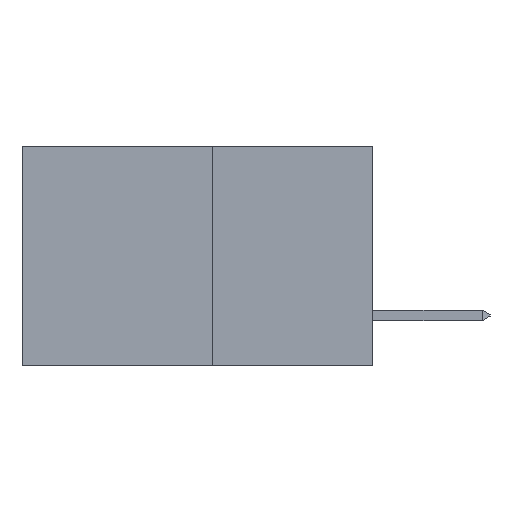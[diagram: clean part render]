
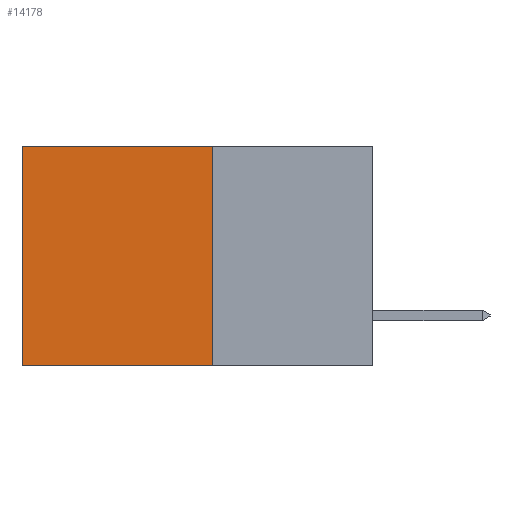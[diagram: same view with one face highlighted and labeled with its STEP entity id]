
A CAD part, left-side view. The second image highlights one B-rep face of the part: STEP entity #14178.
In plain terms, the highlighted planar face has unit normal (-1, 0, 0).
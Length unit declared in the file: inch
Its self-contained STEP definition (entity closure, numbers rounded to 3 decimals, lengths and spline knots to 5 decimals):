
#647 = CARTESIAN_POINT ( 'NONE',  ( 0.277, 0.27, -0.37 ) ) ;
#1127 = DIRECTION ( 'NONE',  ( 0., 0., -1. ) ) ;
#1196 = CARTESIAN_POINT ( 'NONE',  ( 0.277, 0.59, -0.37 ) ) ;
#1388 = VERTEX_POINT ( 'NONE', #10298 ) ;
#2041 = CARTESIAN_POINT ( 'NONE',  ( 0.277, 0.59, -0.37 ) ) ;
#2064 = EDGE_LOOP ( 'NONE', ( #6941, #7075, #2774, #9379 ) ) ;
#2774 = ORIENTED_EDGE ( 'NONE', *, *, #3381, .F. ) ;
#3226 = VERTEX_POINT ( 'NONE', #1196 ) ;
#3381 = EDGE_CURVE ( 'NONE', #1388, #15335, #8486, .T. ) ;
#3581 = DIRECTION ( 'NONE',  ( 0., 0., -1. ) ) ;
#3690 = DIRECTION ( 'NONE',  ( 0., 1., 0. ) ) ;
#3739 = DIRECTION ( 'NONE',  ( 0., 0., -1. ) ) ;
#3917 = VECTOR ( 'NONE', #13736, 39.37008 ) ;
#5325 = LINE ( 'NONE', #15149, #3917 ) ;
#5995 = VECTOR ( 'NONE', #3690, 39.37008 ) ;
#6291 = VERTEX_POINT ( 'NONE', #17651 ) ;
#6637 = EDGE_CURVE ( 'NONE', #6291, #3226, #11202, .T. ) ;
#6914 = LINE ( 'NONE', #14098, #5995 ) ;
#6941 = ORIENTED_EDGE ( 'NONE', *, *, #6637, .T. ) ;
#7075 = ORIENTED_EDGE ( 'NONE', *, *, #7158, .F. ) ;
#7158 = EDGE_CURVE ( 'NONE', #15335, #3226, #5325, .T. ) ;
#7895 = CARTESIAN_POINT ( 'NONE',  ( 0.277, 0.27, -0.37 ) ) ;
#8162 = AXIS2_PLACEMENT_3D ( 'NONE', #647, #12715, #3739 ) ;
#8486 = LINE ( 'NONE', #18847, #11987 ) ;
#9379 = ORIENTED_EDGE ( 'NONE', *, *, #12828, .T. ) ;
#10298 = CARTESIAN_POINT ( 'NONE',  ( 0.277, 0.27, 0. ) ) ;
#10733 = VECTOR ( 'NONE', #3581, 39.37008 ) ;
#11202 = LINE ( 'NONE', #2041, #10733 ) ;
#11987 = VECTOR ( 'NONE', #1127, 39.37008 ) ;
#12715 = DIRECTION ( 'NONE',  ( 1., 0., 0. ) ) ;
#12828 = EDGE_CURVE ( 'NONE', #1388, #6291, #6914, .T. ) ;
#13736 = DIRECTION ( 'NONE',  ( 0., 1., 0. ) ) ;
#14098 = CARTESIAN_POINT ( 'NONE',  ( 0.277, 0.27, 0. ) ) ;
#14178 = ADVANCED_FACE ( 'NONE', ( #18025 ), #17070, .F. ) ;
#15149 = CARTESIAN_POINT ( 'NONE',  ( 0.277, 0.27, -0.37 ) ) ;
#15335 = VERTEX_POINT ( 'NONE', #7895 ) ;
#17070 = PLANE ( 'NONE',  #8162 ) ;
#17651 = CARTESIAN_POINT ( 'NONE',  ( 0.277, 0.59, 0. ) ) ;
#18025 = FACE_OUTER_BOUND ( 'NONE', #2064, .T. ) ;
#18847 = CARTESIAN_POINT ( 'NONE',  ( 0.277, 0.27, -0.37 ) ) ;
